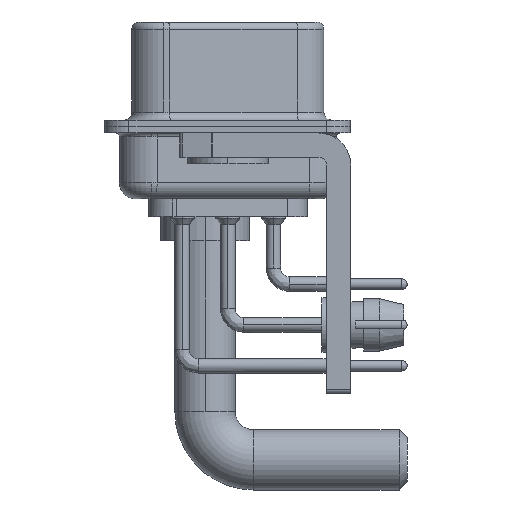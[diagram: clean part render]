
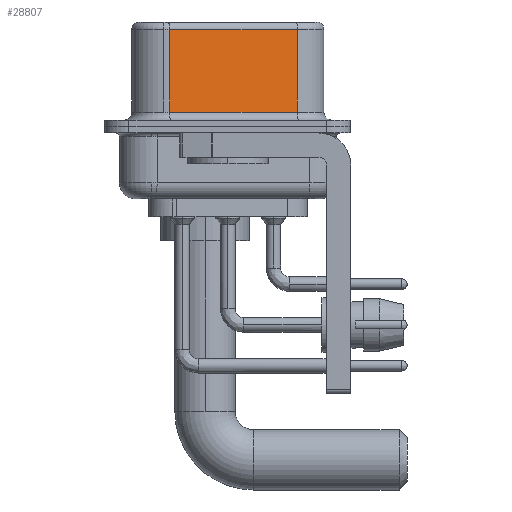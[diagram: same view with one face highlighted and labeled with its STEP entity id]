
A CAD part, left-side view. The second image highlights one B-rep face of the part: STEP entity #28807.
In plain terms, the highlighted planar face has unit normal (-0.985, -0.174, 0).
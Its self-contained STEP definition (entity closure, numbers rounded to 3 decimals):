
#264 = EDGE_CURVE ( 'NONE', #6775, #25225, #22236, .T. ) ;
#1054 = VERTEX_POINT ( 'NONE', #20749 ) ;
#3679 = CARTESIAN_POINT ( 'NONE',  ( 5.132, -4.322, 6.52 ) ) ;
#3828 = FACE_OUTER_BOUND ( 'NONE', #7355, .T. ) ;
#4680 = CARTESIAN_POINT ( 'NONE',  ( 5.132, -4.322, 6.02 ) ) ;
#4789 = CARTESIAN_POINT ( 'NONE',  ( 5.132, -4.322, 0.9 ) ) ;
#6775 = VERTEX_POINT ( 'NONE', #33570 ) ;
#7355 = EDGE_LOOP ( 'NONE', ( #22525, #21556, #28594, #26870 ) ) ;
#7814 = DIRECTION ( 'NONE',  ( 0., 0., -1. ) ) ;
#9980 = LINE ( 'NONE', #25215, #18935 ) ;
#10316 = CARTESIAN_POINT ( 'NONE',  ( 5.132, -4.322, 0.9 ) ) ;
#13194 = VECTOR ( 'NONE', #23241, 1000. ) ;
#15569 = VERTEX_POINT ( 'NONE', #22841 ) ;
#17089 = AXIS2_PLACEMENT_3D ( 'NONE', #30221, #21801, #18673 ) ;
#18330 = VECTOR ( 'NONE', #22049, 1000. ) ;
#18673 = DIRECTION ( 'NONE',  ( -0.174, 0.985, 0. ) ) ;
#18935 = VECTOR ( 'NONE', #7814, 1000. ) ;
#20749 = CARTESIAN_POINT ( 'NONE',  ( 3.73, 3.628, 6.02 ) ) ;
#21454 = LINE ( 'NONE', #3679, #32563 ) ;
#21556 = ORIENTED_EDGE ( 'NONE', *, *, #24883, .T. ) ;
#21801 = DIRECTION ( 'NONE',  ( 0.985, 0.174, 0. ) ) ;
#22049 = DIRECTION ( 'NONE',  ( 0.174, -0.985, 0. ) ) ;
#22236 = LINE ( 'NONE', #10316, #18330 ) ;
#22525 = ORIENTED_EDGE ( 'NONE', *, *, #25236, .F. ) ;
#22841 = CARTESIAN_POINT ( 'NONE',  ( 5.132, -4.322, 6.02 ) ) ;
#23241 = DIRECTION ( 'NONE',  ( -0.174, 0.985, 0. ) ) ;
#24883 = EDGE_CURVE ( 'NONE', #15569, #1054, #26374, .T. ) ;
#25215 = CARTESIAN_POINT ( 'NONE',  ( 3.73, 3.628, 6.52 ) ) ;
#25225 = VERTEX_POINT ( 'NONE', #4789 ) ;
#25236 = EDGE_CURVE ( 'NONE', #15569, #25225, #21454, .T. ) ;
#26374 = LINE ( 'NONE', #4680, #13194 ) ;
#26870 = ORIENTED_EDGE ( 'NONE', *, *, #264, .T. ) ;
#27477 = PLANE ( 'NONE',  #17089 ) ;
#28594 = ORIENTED_EDGE ( 'NONE', *, *, #34165, .T. ) ;
#28807 = ADVANCED_FACE ( 'NONE', ( #3828 ), #27477, .F. ) ;
#30221 = CARTESIAN_POINT ( 'NONE',  ( 5.132, -4.322, 6.52 ) ) ;
#32563 = VECTOR ( 'NONE', #37255, 1000. ) ;
#33570 = CARTESIAN_POINT ( 'NONE',  ( 3.73, 3.628, 0.9 ) ) ;
#34165 = EDGE_CURVE ( 'NONE', #1054, #6775, #9980, .T. ) ;
#37255 = DIRECTION ( 'NONE',  ( 0., 0., -1. ) ) ;
